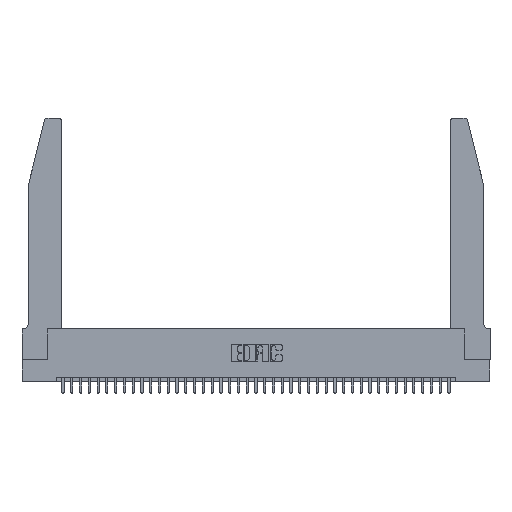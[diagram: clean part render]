
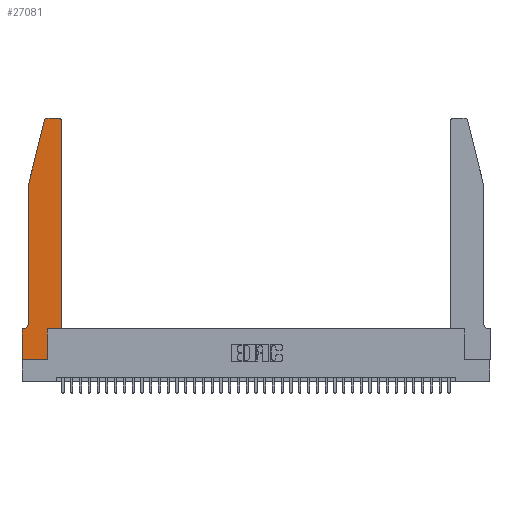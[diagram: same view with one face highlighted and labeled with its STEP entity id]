
A CAD part, top view. The second image highlights one B-rep face of the part: STEP entity #27081.
In plain terms, the highlighted planar face has unit normal (0, 0, 1).
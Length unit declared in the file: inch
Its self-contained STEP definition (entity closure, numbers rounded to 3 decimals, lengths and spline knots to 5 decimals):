
#146 = LINE ( 'NONE', #18558, #7620 ) ;
#654 = VECTOR ( 'NONE', #32626, 39.37008 ) ;
#720 = DIRECTION ( 'NONE',  ( 0., 1., 0. ) ) ;
#914 = DIRECTION ( 'NONE',  ( 1., 0., 0. ) ) ;
#1257 = DIRECTION ( 'NONE',  ( 0., -1., 0. ) ) ;
#1275 = CARTESIAN_POINT ( 'NONE',  ( 0.284, 2.75, 0.37 ) ) ;
#2488 = ORIENTED_EDGE ( 'NONE', *, *, #12179, .T. ) ;
#2798 = VERTEX_POINT ( 'NONE', #38242 ) ;
#3161 = DIRECTION ( 'NONE',  ( 1., 0., 0. ) ) ;
#3656 = VERTEX_POINT ( 'NONE', #36361 ) ;
#3709 = LINE ( 'NONE', #37434, #19052 ) ;
#3931 = FACE_OUTER_BOUND ( 'NONE', #27058, .T. ) ;
#4354 = CARTESIAN_POINT ( 'NONE',  ( 0.0755, 2., 0.37 ) ) ;
#4942 = ORIENTED_EDGE ( 'NONE', *, *, #30119, .T. ) ;
#6112 = EDGE_CURVE ( 'NONE', #9975, #37056, #35261, .T. ) ;
#6225 = CARTESIAN_POINT ( 'NONE',  ( 0.4205, 2.75, 0.37 ) ) ;
#6250 = LINE ( 'NONE', #26440, #39548 ) ;
#6345 = EDGE_CURVE ( 'NONE', #2798, #17044, #28617, .T. ) ;
#6772 = AXIS2_PLACEMENT_3D ( 'NONE', #28426, #10168, #31475 ) ;
#6891 = EDGE_CURVE ( 'NONE', #30386, #3656, #26195, .T. ) ;
#7620 = VECTOR ( 'NONE', #27778, 39.37008 ) ;
#8539 = CIRCLE ( 'NONE', #27967, 0.03 ) ;
#8909 = ORIENTED_EDGE ( 'NONE', *, *, #6891, .T. ) ;
#9568 = VERTEX_POINT ( 'NONE', #30368 ) ;
#9975 = VERTEX_POINT ( 'NONE', #29151 ) ;
#9995 = VERTEX_POINT ( 'NONE', #16902 ) ;
#10168 = DIRECTION ( 'NONE',  ( 0., 0., -1. ) ) ;
#10675 = CARTESIAN_POINT ( 'NONE',  ( 0.0755, 2., 0.37 ) ) ;
#10693 = ORIENTED_EDGE ( 'NONE', *, *, #11897, .T. ) ;
#11251 = DIRECTION ( 'NONE',  ( -1., 0., 0. ) ) ;
#11573 = AXIS2_PLACEMENT_3D ( 'NONE', #30687, #15542, #36762 ) ;
#11753 = CARTESIAN_POINT ( 'NONE',  ( 0., 0., 0.37 ) ) ;
#11897 = EDGE_CURVE ( 'NONE', #3656, #13021, #146, .T. ) ;
#12179 = EDGE_CURVE ( 'NONE', #17044, #30386, #23383, .T. ) ;
#12466 = EDGE_CURVE ( 'NONE', #13021, #9975, #30018, .T. ) ;
#13021 = VERTEX_POINT ( 'NONE', #38378 ) ;
#13148 = EDGE_CURVE ( 'NONE', #9995, #37558, #23309, .T. ) ;
#13333 = CARTESIAN_POINT ( 'NONE',  ( 0.4505, 0.35, 0.37 ) ) ;
#14402 = CARTESIAN_POINT ( 'NONE',  ( 0.2865, 0.35, 0.37 ) ) ;
#14427 = CARTESIAN_POINT ( 'NONE',  ( 0.0755, 0.42, 0.37 ) ) ;
#14793 = DIRECTION ( 'NONE',  ( 0., 0., 1. ) ) ;
#15267 = VECTOR ( 'NONE', #1257, 39.37008 ) ;
#15542 = DIRECTION ( 'NONE',  ( 0., 0., 1. ) ) ;
#15964 = VECTOR ( 'NONE', #914, 39.37008 ) ;
#16289 = DIRECTION ( 'NONE',  ( 0., 0., 1. ) ) ;
#16474 = DIRECTION ( 'NONE',  ( -0.239, -0.971, 0. ) ) ;
#16902 = CARTESIAN_POINT ( 'NONE',  ( 0.4505, 2.72, 0.37 ) ) ;
#17044 = VERTEX_POINT ( 'NONE', #10675 ) ;
#17860 = DIRECTION ( 'NONE',  ( 0., -1., 0. ) ) ;
#18558 = CARTESIAN_POINT ( 'NONE',  ( 0.0755, 0.35, 0.37 ) ) ;
#19052 = VECTOR ( 'NONE', #720, 39.37008 ) ;
#19091 = VECTOR ( 'NONE', #3161, 39.37008 ) ;
#19875 = VERTEX_POINT ( 'NONE', #21970 ) ;
#20106 = ORIENTED_EDGE ( 'NONE', *, *, #37943, .T. ) ;
#20909 = EDGE_CURVE ( 'NONE', #19875, #9995, #3709, .T. ) ;
#21337 = ORIENTED_EDGE ( 'NONE', *, *, #12466, .T. ) ;
#21970 = CARTESIAN_POINT ( 'NONE',  ( 0.4505, 0.35, 0.37 ) ) ;
#23309 = CIRCLE ( 'NONE', #33960, 0.03 ) ;
#23383 = LINE ( 'NONE', #4354, #15267 ) ;
#23434 = ORIENTED_EDGE ( 'NONE', *, *, #20909, .T. ) ;
#24342 = LINE ( 'NONE', #14402, #654 ) ;
#24641 = CARTESIAN_POINT ( 'NONE',  ( 0., 0., 0.37 ) ) ;
#25040 = LINE ( 'NONE', #13333, #15964 ) ;
#26195 = CIRCLE ( 'NONE', #6772, 0.07 ) ;
#26440 = CARTESIAN_POINT ( 'NONE',  ( 0.2605, 2.75, 0.37 ) ) ;
#27058 = EDGE_LOOP ( 'NONE', ( #36034, #4942, #37347, #2488, #8909, #10693, #21337, #28842, #20106, #30233, #23434, #27581 ) ) ;
#27081 = ADVANCED_FACE ( 'NONE', ( #3931 ), #27654, .T. ) ;
#27403 = VERTEX_POINT ( 'NONE', #1275 ) ;
#27581 = ORIENTED_EDGE ( 'NONE', *, *, #13148, .T. ) ;
#27654 = PLANE ( 'NONE',  #11573 ) ;
#27670 = VECTOR ( 'NONE', #16474, 39.37008 ) ;
#27778 = DIRECTION ( 'NONE',  ( -1., 0., 0. ) ) ;
#27912 = CARTESIAN_POINT ( 'NONE',  ( 0.2865, 0., 0.37 ) ) ;
#27967 = AXIS2_PLACEMENT_3D ( 'NONE', #34496, #16289, #37522 ) ;
#28426 = CARTESIAN_POINT ( 'NONE',  ( 0.0055, 0.42, 0.37 ) ) ;
#28617 = LINE ( 'NONE', #31640, #27670 ) ;
#28842 = ORIENTED_EDGE ( 'NONE', *, *, #6112, .T. ) ;
#29151 = CARTESIAN_POINT ( 'NONE',  ( 0., 0., 0.37 ) ) ;
#30018 = LINE ( 'NONE', #11753, #38017 ) ;
#30119 = EDGE_CURVE ( 'NONE', #27403, #2798, #8539, .T. ) ;
#30233 = ORIENTED_EDGE ( 'NONE', *, *, #34190, .T. ) ;
#30368 = CARTESIAN_POINT ( 'NONE',  ( 0.2865, 0.35, 0.37 ) ) ;
#30386 = VERTEX_POINT ( 'NONE', #14427 ) ;
#30687 = CARTESIAN_POINT ( 'NONE',  ( 0., 0.35, 0.37 ) ) ;
#31475 = DIRECTION ( 'NONE',  ( -1., 0., 0. ) ) ;
#31640 = CARTESIAN_POINT ( 'NONE',  ( 0.0755, 2., 0.37 ) ) ;
#32626 = DIRECTION ( 'NONE',  ( 0., 1., 0. ) ) ;
#32993 = CARTESIAN_POINT ( 'NONE',  ( 0.4205, 2.72, 0.37 ) ) ;
#33960 = AXIS2_PLACEMENT_3D ( 'NONE', #32993, #14793, #36018 ) ;
#34190 = EDGE_CURVE ( 'NONE', #9568, #19875, #25040, .T. ) ;
#34496 = CARTESIAN_POINT ( 'NONE',  ( 0.284, 2.72, 0.37 ) ) ;
#35261 = LINE ( 'NONE', #24641, #19091 ) ;
#35345 = EDGE_CURVE ( 'NONE', #37558, #27403, #6250, .T. ) ;
#36018 = DIRECTION ( 'NONE',  ( 1., 0., 0. ) ) ;
#36034 = ORIENTED_EDGE ( 'NONE', *, *, #35345, .T. ) ;
#36361 = CARTESIAN_POINT ( 'NONE',  ( 0.0055, 0.35, 0.37 ) ) ;
#36762 = DIRECTION ( 'NONE',  ( 1., 0., 0. ) ) ;
#37056 = VERTEX_POINT ( 'NONE', #27912 ) ;
#37347 = ORIENTED_EDGE ( 'NONE', *, *, #6345, .T. ) ;
#37434 = CARTESIAN_POINT ( 'NONE',  ( 0.4505, 0.35, 0.37 ) ) ;
#37522 = DIRECTION ( 'NONE',  ( 1., 0., 0. ) ) ;
#37558 = VERTEX_POINT ( 'NONE', #6225 ) ;
#37943 = EDGE_CURVE ( 'NONE', #37056, #9568, #24342, .T. ) ;
#38017 = VECTOR ( 'NONE', #17860, 39.37008 ) ;
#38242 = CARTESIAN_POINT ( 'NONE',  ( 0.25487, 2.72718, 0.37 ) ) ;
#38378 = CARTESIAN_POINT ( 'NONE',  ( 0., 0.35, 0.37 ) ) ;
#39548 = VECTOR ( 'NONE', #11251, 39.37008 ) ;
